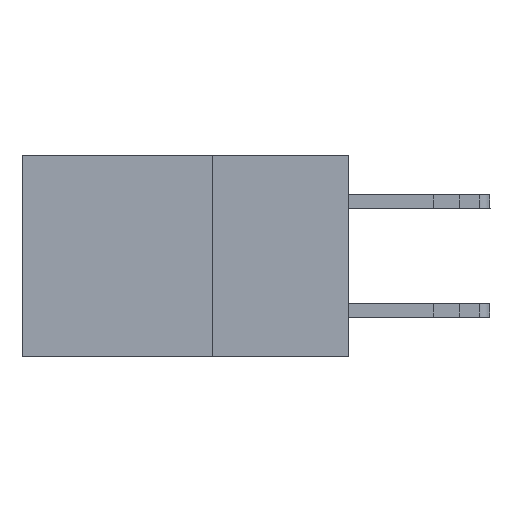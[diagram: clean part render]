
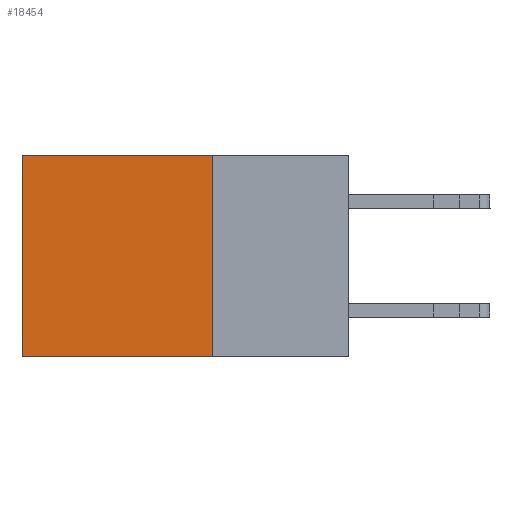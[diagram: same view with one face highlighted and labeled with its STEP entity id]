
A CAD part, left-side view. The second image highlights one B-rep face of the part: STEP entity #18454.
In plain terms, the highlighted planar face has unit normal (-1, 0, 0).
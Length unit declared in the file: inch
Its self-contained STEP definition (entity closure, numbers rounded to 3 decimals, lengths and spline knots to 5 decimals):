
#1073 = FACE_OUTER_BOUND ( 'NONE', #9869, .T. ) ;
#1536 = LINE ( 'NONE', #11358, #10371 ) ;
#1537 = CARTESIAN_POINT ( 'NONE',  ( 0.2615, 0.25, 0. ) ) ;
#2384 = LINE ( 'NONE', #20570, #11786 ) ;
#2419 = ORIENTED_EDGE ( 'NONE', *, *, #23541, .T. ) ;
#3259 = ORIENTED_EDGE ( 'NONE', *, *, #5100, .F. ) ;
#3426 = DIRECTION ( 'NONE',  ( 0., 1., 0. ) ) ;
#4061 = ORIENTED_EDGE ( 'NONE', *, *, #15074, .T. ) ;
#4272 = ORIENTED_EDGE ( 'NONE', *, *, #19863, .F. ) ;
#4920 = VERTEX_POINT ( 'NONE', #12746 ) ;
#5100 = EDGE_CURVE ( 'NONE', #8799, #19525, #1536, .T. ) ;
#6854 = CARTESIAN_POINT ( 'NONE',  ( 0.2615, 0.6, -0.37 ) ) ;
#7520 = DIRECTION ( 'NONE',  ( 0., 0., -1. ) ) ;
#8799 = VERTEX_POINT ( 'NONE', #19066 ) ;
#9869 = EDGE_LOOP ( 'NONE', ( #4061, #4272, #3259, #2419 ) ) ;
#10371 = VECTOR ( 'NONE', #7520, 39.37008 ) ;
#11358 = CARTESIAN_POINT ( 'NONE',  ( 0.2615, 0.25, -0.37 ) ) ;
#11373 = DIRECTION ( 'NONE',  ( 0., 1., 0. ) ) ;
#11786 = VECTOR ( 'NONE', #11373, 39.37008 ) ;
#12746 = CARTESIAN_POINT ( 'NONE',  ( 0.2615, 0.6, 0. ) ) ;
#12880 = DIRECTION ( 'NONE',  ( 0., 0., -1. ) ) ;
#15074 = EDGE_CURVE ( 'NONE', #4920, #20941, #21012, .T. ) ;
#16081 = CARTESIAN_POINT ( 'NONE',  ( 0.2615, 0.25, -0.37 ) ) ;
#16411 = AXIS2_PLACEMENT_3D ( 'NONE', #22072, #23913, #12880 ) ;
#18293 = LINE ( 'NONE', #1537, #18874 ) ;
#18384 = PLANE ( 'NONE',  #16411 ) ;
#18454 = ADVANCED_FACE ( 'NONE', ( #1073 ), #18384, .F. ) ;
#18874 = VECTOR ( 'NONE', #3426, 39.37008 ) ;
#19066 = CARTESIAN_POINT ( 'NONE',  ( 0.2615, 0.25, 0. ) ) ;
#19525 = VERTEX_POINT ( 'NONE', #16081 ) ;
#19863 = EDGE_CURVE ( 'NONE', #19525, #20941, #2384, .T. ) ;
#19900 = CARTESIAN_POINT ( 'NONE',  ( 0.2615, 0.6, -0.37 ) ) ;
#20438 = VECTOR ( 'NONE', #21846, 39.37008 ) ;
#20570 = CARTESIAN_POINT ( 'NONE',  ( 0.2615, 0.25, -0.37 ) ) ;
#20941 = VERTEX_POINT ( 'NONE', #19900 ) ;
#21012 = LINE ( 'NONE', #6854, #20438 ) ;
#21846 = DIRECTION ( 'NONE',  ( 0., 0., -1. ) ) ;
#22072 = CARTESIAN_POINT ( 'NONE',  ( 0.2615, 0.25, -0.37 ) ) ;
#23541 = EDGE_CURVE ( 'NONE', #8799, #4920, #18293, .T. ) ;
#23913 = DIRECTION ( 'NONE',  ( 1., 0., 0. ) ) ;
